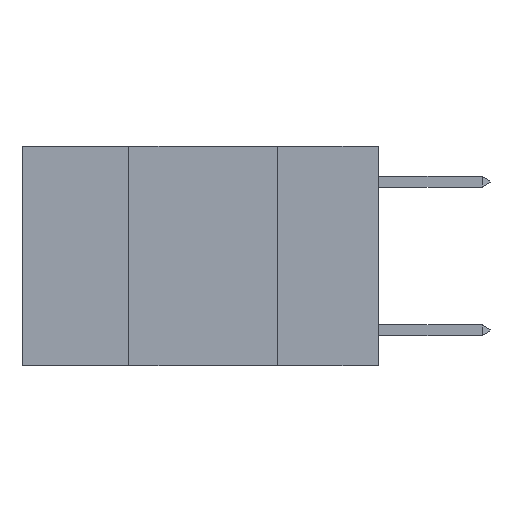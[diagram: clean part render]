
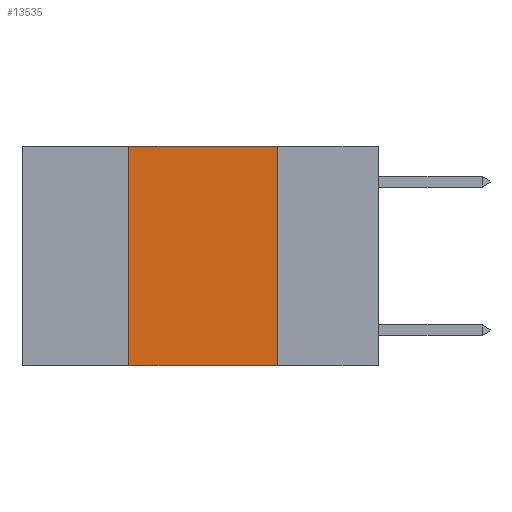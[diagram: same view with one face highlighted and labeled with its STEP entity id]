
A CAD part, left-side view. The second image highlights one B-rep face of the part: STEP entity #13535.
In plain terms, the highlighted planar face has unit normal (-1, 0, 0).
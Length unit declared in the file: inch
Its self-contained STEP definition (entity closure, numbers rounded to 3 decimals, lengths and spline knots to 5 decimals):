
#46 = LINE ( 'NONE', #13524, #10561 ) ;
#775 = CARTESIAN_POINT ( 'NONE',  ( 0., 0.6, 0. ) ) ;
#2163 = EDGE_CURVE ( 'NONE', #11938, #13382, #12721, .T. ) ;
#2286 = VECTOR ( 'NONE', #4021, 39.37008 ) ;
#2373 = VERTEX_POINT ( 'NONE', #4255 ) ;
#3044 = ORIENTED_EDGE ( 'NONE', *, *, #3757, .F. ) ;
#3123 = DIRECTION ( 'NONE',  ( 1., 0., 0. ) ) ;
#3284 = ORIENTED_EDGE ( 'NONE', *, *, #13312, .T. ) ;
#3539 = CARTESIAN_POINT ( 'NONE',  ( 0., 0.42, -0.37 ) ) ;
#3652 = ORIENTED_EDGE ( 'NONE', *, *, #2163, .F. ) ;
#3747 = DIRECTION ( 'NONE',  ( 0., 0., -1. ) ) ;
#3757 = EDGE_CURVE ( 'NONE', #13382, #4665, #46, .T. ) ;
#3985 = CARTESIAN_POINT ( 'NONE',  ( 0., 0.17, 0. ) ) ;
#4021 = DIRECTION ( 'NONE',  ( 0., 0., 1. ) ) ;
#4088 = CARTESIAN_POINT ( 'NONE',  ( 0., 0.42, 0. ) ) ;
#4255 = CARTESIAN_POINT ( 'NONE',  ( 0., 0.17, -0.37 ) ) ;
#4258 = FACE_OUTER_BOUND ( 'NONE', #11283, .T. ) ;
#4336 = PLANE ( 'NONE',  #4545 ) ;
#4413 = EDGE_CURVE ( 'NONE', #4665, #2373, #5269, .T. ) ;
#4545 = AXIS2_PLACEMENT_3D ( 'NONE', #775, #3123, #14104 ) ;
#4665 = VERTEX_POINT ( 'NONE', #15813 ) ;
#4708 = ORIENTED_EDGE ( 'NONE', *, *, #4413, .F. ) ;
#4807 = VECTOR ( 'NONE', #11579, 39.37008 ) ;
#5269 = LINE ( 'NONE', #3985, #8767 ) ;
#8767 = VECTOR ( 'NONE', #3747, 39.37008 ) ;
#8974 = CARTESIAN_POINT ( 'NONE',  ( 0., 0.6, -0.37 ) ) ;
#10561 = VECTOR ( 'NONE', #13447, 39.37008 ) ;
#11283 = EDGE_LOOP ( 'NONE', ( #4708, #3044, #3652, #3284 ) ) ;
#11579 = DIRECTION ( 'NONE',  ( 0., -1., 0. ) ) ;
#11938 = VERTEX_POINT ( 'NONE', #3539 ) ;
#12721 = LINE ( 'NONE', #4088, #2286 ) ;
#13312 = EDGE_CURVE ( 'NONE', #11938, #2373, #15207, .T. ) ;
#13382 = VERTEX_POINT ( 'NONE', #15055 ) ;
#13447 = DIRECTION ( 'NONE',  ( 0., -1., 0. ) ) ;
#13524 = CARTESIAN_POINT ( 'NONE',  ( 0., 0.6, 0. ) ) ;
#13535 = ADVANCED_FACE ( 'NONE', ( #4258 ), #4336, .F. ) ;
#14104 = DIRECTION ( 'NONE',  ( 0., 0., -1. ) ) ;
#15055 = CARTESIAN_POINT ( 'NONE',  ( 0., 0.42, 0. ) ) ;
#15207 = LINE ( 'NONE', #8974, #4807 ) ;
#15813 = CARTESIAN_POINT ( 'NONE',  ( 0., 0.17, 0. ) ) ;
